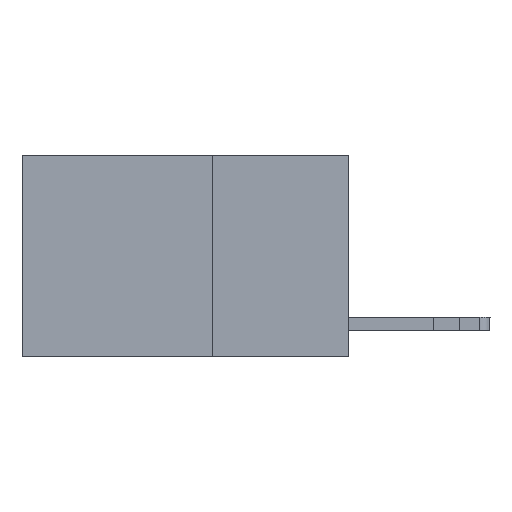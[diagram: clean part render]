
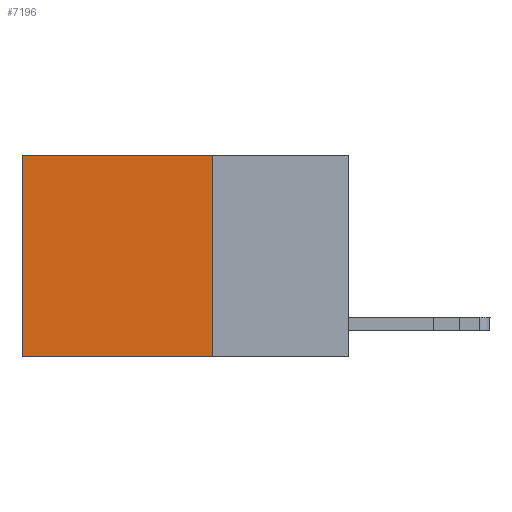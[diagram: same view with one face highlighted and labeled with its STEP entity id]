
A CAD part, left-side view. The second image highlights one B-rep face of the part: STEP entity #7196.
In plain terms, the highlighted planar face has unit normal (-1, 0, 0).
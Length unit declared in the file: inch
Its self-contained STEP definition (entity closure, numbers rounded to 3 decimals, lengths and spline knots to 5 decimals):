
#221 = VECTOR ( 'NONE', #1407, 39.37008 ) ;
#474 = PLANE ( 'NONE',  #2776 ) ;
#588 = CARTESIAN_POINT ( 'NONE',  ( 0.2625, 0.25, -0.37 ) ) ;
#1407 = DIRECTION ( 'NONE',  ( 0., 1., 0. ) ) ;
#2661 = CARTESIAN_POINT ( 'NONE',  ( 0.2625, 0.6, 0. ) ) ;
#2776 = AXIS2_PLACEMENT_3D ( 'NONE', #16935, #6481, #17003 ) ;
#3948 = EDGE_LOOP ( 'NONE', ( #8427, #12190, #11121, #8693 ) ) ;
#4341 = CARTESIAN_POINT ( 'NONE',  ( 0.2625, 0.25, -0.37 ) ) ;
#4423 = VERTEX_POINT ( 'NONE', #5197 ) ;
#4614 = EDGE_CURVE ( 'NONE', #13981, #11074, #7860, .T. ) ;
#5197 = CARTESIAN_POINT ( 'NONE',  ( 0.2625, 0.6, 0. ) ) ;
#6481 = DIRECTION ( 'NONE',  ( 1., 0., 0. ) ) ;
#6571 = FACE_OUTER_BOUND ( 'NONE', #3948, .T. ) ;
#7150 = LINE ( 'NONE', #588, #10736 ) ;
#7196 = ADVANCED_FACE ( 'NONE', ( #6571 ), #474, .F. ) ;
#7860 = LINE ( 'NONE', #17625, #19349 ) ;
#8427 = ORIENTED_EDGE ( 'NONE', *, *, #17707, .T. ) ;
#8693 = ORIENTED_EDGE ( 'NONE', *, *, #15909, .T. ) ;
#10440 = CARTESIAN_POINT ( 'NONE',  ( 0.2625, 0.25, 0. ) ) ;
#10736 = VECTOR ( 'NONE', #12621, 39.37008 ) ;
#10754 = VECTOR ( 'NONE', #17708, 39.37008 ) ;
#11074 = VERTEX_POINT ( 'NONE', #4341 ) ;
#11121 = ORIENTED_EDGE ( 'NONE', *, *, #4614, .F. ) ;
#11729 = CARTESIAN_POINT ( 'NONE',  ( 0.2625, 0.25, 0. ) ) ;
#12190 = ORIENTED_EDGE ( 'NONE', *, *, #17950, .F. ) ;
#12621 = DIRECTION ( 'NONE',  ( 0., 1., 0. ) ) ;
#13233 = VERTEX_POINT ( 'NONE', #18735 ) ;
#13981 = VERTEX_POINT ( 'NONE', #11729 ) ;
#14777 = LINE ( 'NONE', #10440, #221 ) ;
#15909 = EDGE_CURVE ( 'NONE', #13981, #4423, #14777, .T. ) ;
#16130 = DIRECTION ( 'NONE',  ( 0., 0., -1. ) ) ;
#16935 = CARTESIAN_POINT ( 'NONE',  ( 0.2625, 0.25, 0. ) ) ;
#17003 = DIRECTION ( 'NONE',  ( 0., 0., -1. ) ) ;
#17625 = CARTESIAN_POINT ( 'NONE',  ( 0.2625, 0.25, 0. ) ) ;
#17707 = EDGE_CURVE ( 'NONE', #4423, #13233, #18691, .T. ) ;
#17708 = DIRECTION ( 'NONE',  ( 0., 0., -1. ) ) ;
#17950 = EDGE_CURVE ( 'NONE', #11074, #13233, #7150, .T. ) ;
#18691 = LINE ( 'NONE', #2661, #10754 ) ;
#18735 = CARTESIAN_POINT ( 'NONE',  ( 0.2625, 0.6, -0.37 ) ) ;
#19349 = VECTOR ( 'NONE', #16130, 39.37008 ) ;
